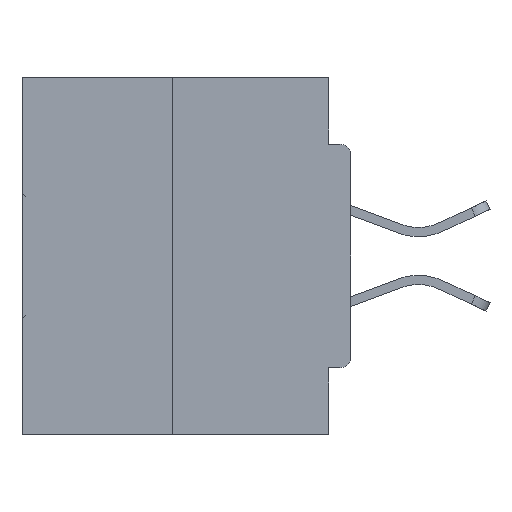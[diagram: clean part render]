
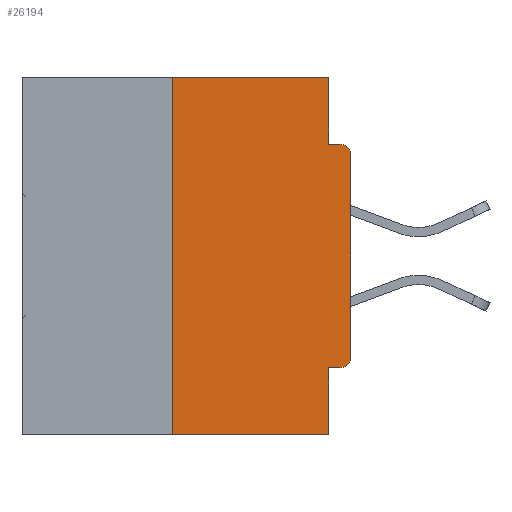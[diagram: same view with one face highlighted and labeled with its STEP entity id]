
A CAD part, left-side view. The second image highlights one B-rep face of the part: STEP entity #26194.
In plain terms, the highlighted planar face has unit normal (-1, 0, 0).
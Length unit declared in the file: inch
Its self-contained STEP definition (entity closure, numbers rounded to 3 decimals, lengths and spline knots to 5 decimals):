
#45 = CIRCLE ( 'NONE', #11217, 0.015 ) ;
#810 = CARTESIAN_POINT ( 'NONE',  ( 0., 0., -0.3915 ) ) ;
#1427 = ORIENTED_EDGE ( 'NONE', *, *, #25612, .F. ) ;
#1984 = DIRECTION ( 'NONE',  ( 0., 0., 1. ) ) ;
#2162 = LINE ( 'NONE', #15498, #39588 ) ;
#2319 = CARTESIAN_POINT ( 'NONE',  ( 0., 0.031, 0. ) ) ;
#2353 = VECTOR ( 'NONE', #33858, 39.37008 ) ;
#2589 = EDGE_CURVE ( 'NONE', #27592, #7001, #35782, .T. ) ;
#3556 = CARTESIAN_POINT ( 'NONE',  ( 0., 0.031, -0.4065 ) ) ;
#3706 = LINE ( 'NONE', #7428, #21761 ) ;
#3785 = LINE ( 'NONE', #17116, #25140 ) ;
#4044 = EDGE_CURVE ( 'NONE', #32489, #8003, #14115, .T. ) ;
#4231 = EDGE_CURVE ( 'NONE', #40974, #21923, #22379, .T. ) ;
#6198 = ORIENTED_EDGE ( 'NONE', *, *, #27299, .T. ) ;
#7001 = VERTEX_POINT ( 'NONE', #42662 ) ;
#7428 = CARTESIAN_POINT ( 'NONE',  ( 0., 0.031, -0.5 ) ) ;
#8003 = VERTEX_POINT ( 'NONE', #40742 ) ;
#8330 = VERTEX_POINT ( 'NONE', #35650 ) ;
#9293 = CARTESIAN_POINT ( 'NONE',  ( 0., 0.25, 0. ) ) ;
#9301 = DIRECTION ( 'NONE',  ( 0., 0., -1. ) ) ;
#11217 = AXIS2_PLACEMENT_3D ( 'NONE', #15843, #12557, #9301 ) ;
#11409 = ORIENTED_EDGE ( 'NONE', *, *, #23613, .T. ) ;
#11643 = VECTOR ( 'NONE', #38391, 39.37008 ) ;
#12557 = DIRECTION ( 'NONE',  ( -1., 0., 0. ) ) ;
#12828 = CARTESIAN_POINT ( 'NONE',  ( 0., 0.031, 0. ) ) ;
#13530 = LINE ( 'NONE', #23781, #2353 ) ;
#14115 = LINE ( 'NONE', #20651, #19293 ) ;
#14116 = VERTEX_POINT ( 'NONE', #9293 ) ;
#14450 = CARTESIAN_POINT ( 'NONE',  ( 0., 0.015, -0.3915 ) ) ;
#14835 = CARTESIAN_POINT ( 'NONE',  ( 0., 0.25, -0.5 ) ) ;
#15498 = CARTESIAN_POINT ( 'NONE',  ( 0., 0.46, 0. ) ) ;
#15843 = CARTESIAN_POINT ( 'NONE',  ( 0., 0.015, -0.1085 ) ) ;
#17116 = CARTESIAN_POINT ( 'NONE',  ( 0., 0., -0.0935 ) ) ;
#17132 = EDGE_CURVE ( 'NONE', #7001, #8330, #3785, .T. ) ;
#17181 = ORIENTED_EDGE ( 'NONE', *, *, #17653, .F. ) ;
#17248 = DIRECTION ( 'NONE',  ( 0., 0., -1. ) ) ;
#17653 = EDGE_CURVE ( 'NONE', #14116, #27592, #2162, .T. ) ;
#18460 = CARTESIAN_POINT ( 'NONE',  ( 0., 0., -0.4065 ) ) ;
#19293 = VECTOR ( 'NONE', #34229, 39.37008 ) ;
#20542 = VECTOR ( 'NONE', #28989, 39.37008 ) ;
#20651 = CARTESIAN_POINT ( 'NONE',  ( 0., 0., 0. ) ) ;
#21404 = DIRECTION ( 'NONE',  ( 0., -1., 0. ) ) ;
#21551 = DIRECTION ( 'NONE',  ( 1., 0., 0. ) ) ;
#21681 = ORIENTED_EDGE ( 'NONE', *, *, #36293, .F. ) ;
#21761 = VECTOR ( 'NONE', #17248, 39.37008 ) ;
#21923 = VERTEX_POINT ( 'NONE', #3556 ) ;
#22379 = LINE ( 'NONE', #18460, #11643 ) ;
#22693 = VERTEX_POINT ( 'NONE', #35192 ) ;
#23567 = ORIENTED_EDGE ( 'NONE', *, *, #2589, .F. ) ;
#23613 = EDGE_CURVE ( 'NONE', #8003, #8330, #45, .T. ) ;
#23781 = CARTESIAN_POINT ( 'NONE',  ( 0., 0.46, -0.5 ) ) ;
#24636 = CARTESIAN_POINT ( 'NONE',  ( 0., 0.46, 0. ) ) ;
#24705 = ORIENTED_EDGE ( 'NONE', *, *, #4044, .T. ) ;
#25140 = VECTOR ( 'NONE', #33955, 39.37008 ) ;
#25612 = EDGE_CURVE ( 'NONE', #21923, #22693, #3706, .T. ) ;
#26194 = ADVANCED_FACE ( 'NONE', ( #35122 ), #34694, .F. ) ;
#27152 = ORIENTED_EDGE ( 'NONE', *, *, #17132, .F. ) ;
#27299 = EDGE_CURVE ( 'NONE', #33906, #22693, #13530, .T. ) ;
#27592 = VERTEX_POINT ( 'NONE', #12828 ) ;
#28006 = LINE ( 'NONE', #31944, #42409 ) ;
#28989 = DIRECTION ( 'NONE',  ( 0., 0., -1. ) ) ;
#31611 = ORIENTED_EDGE ( 'NONE', *, *, #4231, .F. ) ;
#31944 = CARTESIAN_POINT ( 'NONE',  ( 0., 0.25, 0. ) ) ;
#32219 = AXIS2_PLACEMENT_3D ( 'NONE', #14450, #38081, #40943 ) ;
#32489 = VERTEX_POINT ( 'NONE', #810 ) ;
#32927 = CIRCLE ( 'NONE', #32219, 0.015 ) ;
#33858 = DIRECTION ( 'NONE',  ( 0., -1., 0. ) ) ;
#33906 = VERTEX_POINT ( 'NONE', #14835 ) ;
#33955 = DIRECTION ( 'NONE',  ( 0., -1., 0. ) ) ;
#34229 = DIRECTION ( 'NONE',  ( 0., 0., 1. ) ) ;
#34694 = PLANE ( 'NONE',  #37218 ) ;
#35122 = FACE_OUTER_BOUND ( 'NONE', #36709, .T. ) ;
#35192 = CARTESIAN_POINT ( 'NONE',  ( 0., 0.031, -0.5 ) ) ;
#35312 = CARTESIAN_POINT ( 'NONE',  ( 0., 0.015, -0.4065 ) ) ;
#35554 = DIRECTION ( 'NONE',  ( 0., 0., -1. ) ) ;
#35650 = CARTESIAN_POINT ( 'NONE',  ( 0., 0.015, -0.0935 ) ) ;
#35782 = LINE ( 'NONE', #2319, #20542 ) ;
#36293 = EDGE_CURVE ( 'NONE', #33906, #14116, #28006, .T. ) ;
#36709 = EDGE_LOOP ( 'NONE', ( #17181, #21681, #6198, #1427, #31611, #41084, #24705, #11409, #27152, #23567 ) ) ;
#37218 = AXIS2_PLACEMENT_3D ( 'NONE', #24636, #21551, #35554 ) ;
#38081 = DIRECTION ( 'NONE',  ( -1., 0., 0. ) ) ;
#38391 = DIRECTION ( 'NONE',  ( 0., 1., 0. ) ) ;
#39588 = VECTOR ( 'NONE', #21404, 39.37008 ) ;
#40742 = CARTESIAN_POINT ( 'NONE',  ( 0., 0., -0.1085 ) ) ;
#40943 = DIRECTION ( 'NONE',  ( 0., 0., -1. ) ) ;
#40974 = VERTEX_POINT ( 'NONE', #35312 ) ;
#41084 = ORIENTED_EDGE ( 'NONE', *, *, #42851, .T. ) ;
#42409 = VECTOR ( 'NONE', #1984, 39.37008 ) ;
#42662 = CARTESIAN_POINT ( 'NONE',  ( 0., 0.031, -0.0935 ) ) ;
#42851 = EDGE_CURVE ( 'NONE', #40974, #32489, #32927, .T. ) ;
